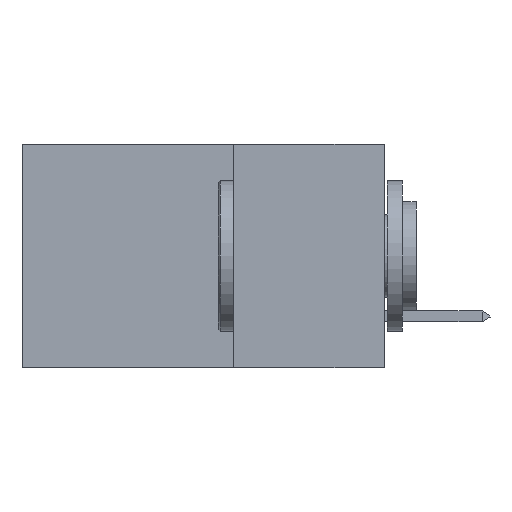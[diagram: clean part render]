
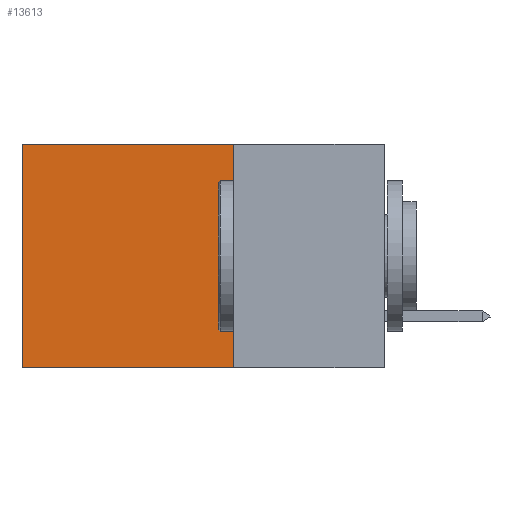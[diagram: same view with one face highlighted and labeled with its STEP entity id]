
A CAD part, left-side view. The second image highlights one B-rep face of the part: STEP entity #13613.
In plain terms, the highlighted planar face has unit normal (-1, 0, 0).
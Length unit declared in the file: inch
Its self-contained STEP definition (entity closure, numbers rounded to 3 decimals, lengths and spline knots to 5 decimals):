
#471 = VERTEX_POINT ( 'NONE', #5507 ) ;
#1165 = EDGE_CURVE ( 'NONE', #6351, #2517, #6262, .T. ) ;
#1305 = DIRECTION ( 'NONE',  ( 0., 1., 0. ) ) ;
#2196 = VECTOR ( 'NONE', #3901, 39.37008 ) ;
#2280 = PLANE ( 'NONE',  #3671 ) ;
#2517 = VERTEX_POINT ( 'NONE', #22581 ) ;
#3671 = AXIS2_PLACEMENT_3D ( 'NONE', #19310, #19397, #21225 ) ;
#3839 = LINE ( 'NONE', #7805, #21056 ) ;
#3901 = DIRECTION ( 'NONE',  ( 0., 1., 0. ) ) ;
#4335 = ORIENTED_EDGE ( 'NONE', *, *, #15170, .F. ) ;
#4360 = VERTEX_POINT ( 'NONE', #11344 ) ;
#4538 = EDGE_LOOP ( 'NONE', ( #22917, #4335, #9427, #11102 ) ) ;
#5507 = CARTESIAN_POINT ( 'NONE',  ( 0.2875, 0.6, -0.37 ) ) ;
#6262 = LINE ( 'NONE', #20574, #2196 ) ;
#6351 = VERTEX_POINT ( 'NONE', #7953 ) ;
#7805 = CARTESIAN_POINT ( 'NONE',  ( 0.2875, 0.6, 0. ) ) ;
#7953 = CARTESIAN_POINT ( 'NONE',  ( 0.2875, 0.25, 0. ) ) ;
#8114 = EDGE_CURVE ( 'NONE', #6351, #4360, #8579, .T. ) ;
#8579 = LINE ( 'NONE', #14767, #18867 ) ;
#8992 = DIRECTION ( 'NONE',  ( 0., 0., -1. ) ) ;
#9427 = ORIENTED_EDGE ( 'NONE', *, *, #8114, .F. ) ;
#11102 = ORIENTED_EDGE ( 'NONE', *, *, #1165, .T. ) ;
#11344 = CARTESIAN_POINT ( 'NONE',  ( 0.2875, 0.25, -0.37 ) ) ;
#13613 = ADVANCED_FACE ( 'NONE', ( #18591 ), #2280, .F. ) ;
#14113 = CARTESIAN_POINT ( 'NONE',  ( 0.2875, 0.25, -0.37 ) ) ;
#14767 = CARTESIAN_POINT ( 'NONE',  ( 0.2875, 0.25, 0. ) ) ;
#15170 = EDGE_CURVE ( 'NONE', #4360, #471, #22199, .T. ) ;
#15968 = VECTOR ( 'NONE', #1305, 39.37008 ) ;
#17290 = DIRECTION ( 'NONE',  ( 0., 0., -1. ) ) ;
#17428 = EDGE_CURVE ( 'NONE', #2517, #471, #3839, .T. ) ;
#18591 = FACE_OUTER_BOUND ( 'NONE', #4538, .T. ) ;
#18867 = VECTOR ( 'NONE', #8992, 39.37008 ) ;
#19310 = CARTESIAN_POINT ( 'NONE',  ( 0.2875, 0.25, 0. ) ) ;
#19397 = DIRECTION ( 'NONE',  ( 1., 0., 0. ) ) ;
#20574 = CARTESIAN_POINT ( 'NONE',  ( 0.2875, 0.25, 0. ) ) ;
#21056 = VECTOR ( 'NONE', #17290, 39.37008 ) ;
#21225 = DIRECTION ( 'NONE',  ( 0., 0., -1. ) ) ;
#22199 = LINE ( 'NONE', #14113, #15968 ) ;
#22581 = CARTESIAN_POINT ( 'NONE',  ( 0.2875, 0.6, 0. ) ) ;
#22917 = ORIENTED_EDGE ( 'NONE', *, *, #17428, .T. ) ;
